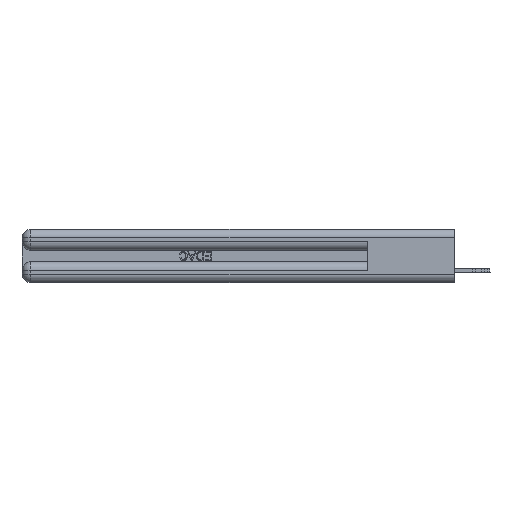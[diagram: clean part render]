
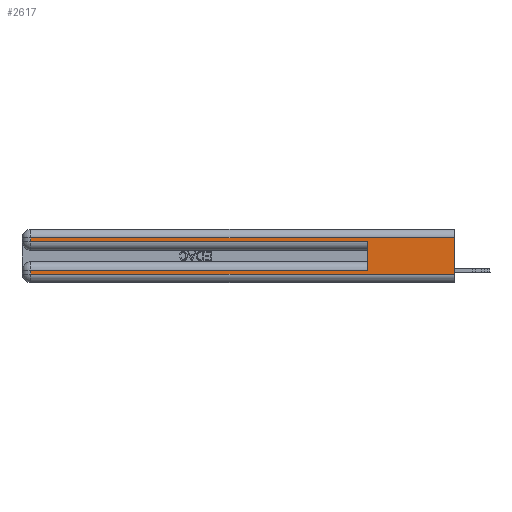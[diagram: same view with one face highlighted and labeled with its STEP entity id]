
A CAD part, left-side view. The second image highlights one B-rep face of the part: STEP entity #2617.
In plain terms, the highlighted planar face has unit normal (-1, 0, 0).
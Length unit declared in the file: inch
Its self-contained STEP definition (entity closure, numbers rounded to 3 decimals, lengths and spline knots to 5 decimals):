
#75 = CARTESIAN_POINT ( 'NONE',  ( 0., 0., 0.285 ) ) ;
#802 = CARTESIAN_POINT ( 'NONE',  ( 0., 0.6, 0.145 ) ) ;
#2149 = VERTEX_POINT ( 'NONE', #40339 ) ;
#2521 = EDGE_CURVE ( 'NONE', #4801, #45261, #36702, .T. ) ;
#2617 = ADVANCED_FACE ( 'NONE', ( #20991 ), #4288, .F. ) ;
#2825 = EDGE_CURVE ( 'NONE', #48021, #19619, #30424, .T. ) ;
#3933 = VECTOR ( 'NONE', #9969, 39.37008 ) ;
#4288 = PLANE ( 'NONE',  #22850 ) ;
#4367 = DIRECTION ( 'NONE',  ( 0., 1., 0. ) ) ;
#4801 = VERTEX_POINT ( 'NONE', #47613 ) ;
#4973 = VECTOR ( 'NONE', #32073, 39.37008 ) ;
#7061 = VECTOR ( 'NONE', #4367, 39.37008 ) ;
#7807 = ORIENTED_EDGE ( 'NONE', *, *, #2825, .T. ) ;
#9969 = DIRECTION ( 'NONE',  ( 0., 0., 1. ) ) ;
#10769 = DIRECTION ( 'NONE',  ( 1., 0., 0. ) ) ;
#11519 = CARTESIAN_POINT ( 'NONE',  ( 0., 0., 0.06 ) ) ;
#11817 = LINE ( 'NONE', #75, #34351 ) ;
#11908 = DIRECTION ( 'NONE',  ( 0., 1., 0. ) ) ;
#12560 = CARTESIAN_POINT ( 'NONE',  ( 0., 0., 0.085 ) ) ;
#12861 = VECTOR ( 'NONE', #50131, 39.37008 ) ;
#15334 = VECTOR ( 'NONE', #11908, 39.37008 ) ;
#15753 = LINE ( 'NONE', #44083, #4973 ) ;
#18025 = VECTOR ( 'NONE', #46131, 39.37008 ) ;
#19619 = VERTEX_POINT ( 'NONE', #38251 ) ;
#19827 = EDGE_CURVE ( 'NONE', #35001, #45261, #40679, .T. ) ;
#20227 = CARTESIAN_POINT ( 'NONE',  ( 0., 0.6, 0.085 ) ) ;
#20991 = FACE_OUTER_BOUND ( 'NONE', #47877, .T. ) ;
#22850 = AXIS2_PLACEMENT_3D ( 'NONE', #50146, #10769, #26882 ) ;
#23585 = VECTOR ( 'NONE', #33283, 39.37008 ) ;
#23973 = LINE ( 'NONE', #36771, #7061 ) ;
#26781 = ORIENTED_EDGE ( 'NONE', *, *, #43737, .T. ) ;
#26882 = DIRECTION ( 'NONE',  ( 0., 0., -1. ) ) ;
#28083 = CARTESIAN_POINT ( 'NONE',  ( 0., 2.94, 0.085 ) ) ;
#28200 = CARTESIAN_POINT ( 'NONE',  ( 0., 2.94, 0.31 ) ) ;
#28609 = DIRECTION ( 'NONE',  ( 0., -1., 0. ) ) ;
#28990 = EDGE_CURVE ( 'NONE', #37706, #2149, #32151, .T. ) ;
#29805 = CARTESIAN_POINT ( 'NONE',  ( 0., 0., 0.06 ) ) ;
#30424 = LINE ( 'NONE', #41581, #23585 ) ;
#31094 = CARTESIAN_POINT ( 'NONE',  ( 0., 0., 0.31 ) ) ;
#32073 = DIRECTION ( 'NONE',  ( 0., 0., -1. ) ) ;
#32151 = LINE ( 'NONE', #802, #3933 ) ;
#32375 = ORIENTED_EDGE ( 'NONE', *, *, #19827, .F. ) ;
#33283 = DIRECTION ( 'NONE',  ( 0., 0., -1. ) ) ;
#33650 = ORIENTED_EDGE ( 'NONE', *, *, #28990, .F. ) ;
#34351 = VECTOR ( 'NONE', #28609, 39.37008 ) ;
#34762 = LINE ( 'NONE', #12560, #15334 ) ;
#35001 = VERTEX_POINT ( 'NONE', #31094 ) ;
#36177 = ORIENTED_EDGE ( 'NONE', *, *, #38738, .T. ) ;
#36702 = LINE ( 'NONE', #29805, #12861 ) ;
#36771 = CARTESIAN_POINT ( 'NONE',  ( 0., 0., 0.31 ) ) ;
#37706 = VERTEX_POINT ( 'NONE', #20227 ) ;
#38251 = CARTESIAN_POINT ( 'NONE',  ( 0., 2.94, 0.285 ) ) ;
#38738 = EDGE_CURVE ( 'NONE', #35001, #48021, #23973, .T. ) ;
#40339 = CARTESIAN_POINT ( 'NONE',  ( 0., 0.6, 0.285 ) ) ;
#40679 = LINE ( 'NONE', #49881, #18025 ) ;
#41581 = CARTESIAN_POINT ( 'NONE',  ( 0., 2.94, 0.37 ) ) ;
#43737 = EDGE_CURVE ( 'NONE', #19619, #2149, #11817, .T. ) ;
#43845 = ORIENTED_EDGE ( 'NONE', *, *, #50790, .T. ) ;
#43981 = ORIENTED_EDGE ( 'NONE', *, *, #2521, .T. ) ;
#44083 = CARTESIAN_POINT ( 'NONE',  ( 0., 2.94, 0.37 ) ) ;
#44300 = VERTEX_POINT ( 'NONE', #28083 ) ;
#45261 = VERTEX_POINT ( 'NONE', #11519 ) ;
#46131 = DIRECTION ( 'NONE',  ( 0., 0., -1. ) ) ;
#47613 = CARTESIAN_POINT ( 'NONE',  ( 0., 2.94, 0.06 ) ) ;
#47877 = EDGE_LOOP ( 'NONE', ( #32375, #36177, #7807, #26781, #33650, #49102, #43845, #43981 ) ) ;
#48021 = VERTEX_POINT ( 'NONE', #28200 ) ;
#48040 = EDGE_CURVE ( 'NONE', #37706, #44300, #34762, .T. ) ;
#49102 = ORIENTED_EDGE ( 'NONE', *, *, #48040, .T. ) ;
#49881 = CARTESIAN_POINT ( 'NONE',  ( 0., 0., 0.37 ) ) ;
#50131 = DIRECTION ( 'NONE',  ( 0., -1., 0. ) ) ;
#50146 = CARTESIAN_POINT ( 'NONE',  ( 0., 0., 0.37 ) ) ;
#50790 = EDGE_CURVE ( 'NONE', #44300, #4801, #15753, .T. ) ;
